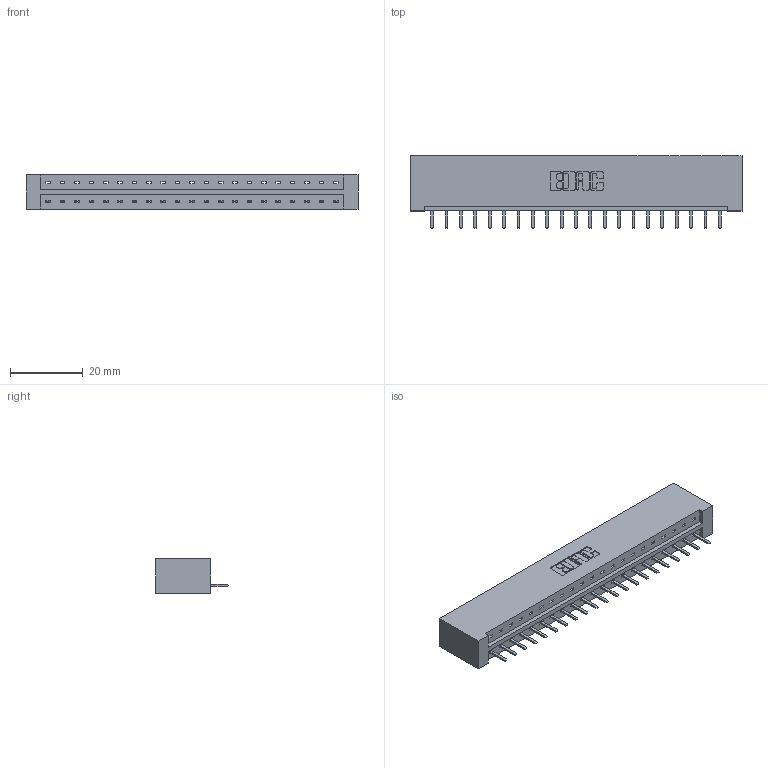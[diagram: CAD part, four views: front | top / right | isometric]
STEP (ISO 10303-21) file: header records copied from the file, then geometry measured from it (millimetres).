
FILE_DESCRIPTION (( 'STEP AP203' ), '1' );
FILE_NAME ('333-021-520-101.STEP', '2018-08-02T00:52:08', ( '' ), ( '' ), 'SwSTEP 2.0', 'SolidWorks 2016', '' );
FILE_SCHEMA (( 'CONFIG_CONTROL_DESIGN' ));
Length unit declared in the file: inch
Products named in the file (3): 333 Part_Lugless; 345-292-001_345-293-120; 333-021-520-101
Assembly tree (22 placements, depth 2):
  333-021-520-101
    333 Part_Lugless
    345-292-001_345-293-120  x21
Bounding box: 91.47 x 20.02 x 9.4 mm (x, y, z)
Volume: 9575.7 mm3; surface area: 9967.9 mm2
Topology: 22 solids, 22 shells, 1408 faces, 4151 edges, 2710 vertices
Faces by surface type: plane 990, cylinder 418
Entity records: 15391 total; most frequent: CARTESIAN_POINT 2677, ORIENTED_EDGE 2622, DIRECTION 2281, EDGE_CURVE 1311, VECTOR 1187, LINE 1187, VERTEX_POINT 870, AXIS2_PLACEMENT_3D 547
